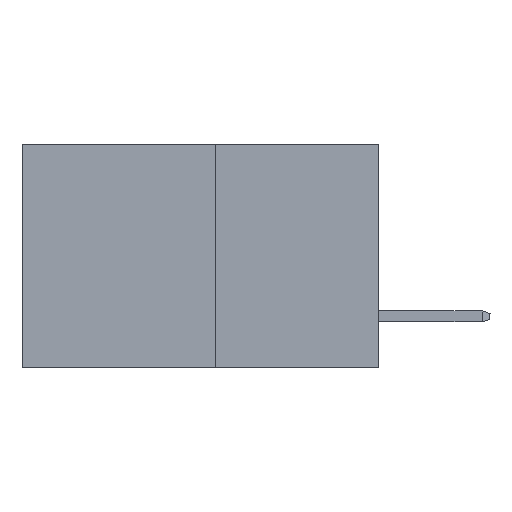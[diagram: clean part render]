
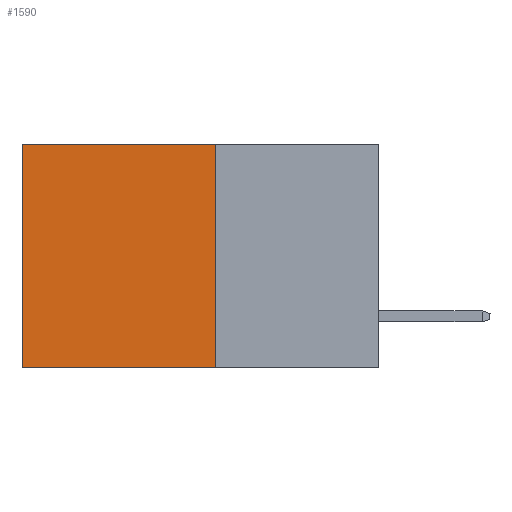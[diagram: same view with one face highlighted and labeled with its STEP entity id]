
A CAD part, left-side view. The second image highlights one B-rep face of the part: STEP entity #1590.
In plain terms, the highlighted planar face has unit normal (-1, 0, 0).
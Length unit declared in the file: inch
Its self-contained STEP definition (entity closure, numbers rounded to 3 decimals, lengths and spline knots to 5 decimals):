
#270 = EDGE_LOOP ( 'NONE', ( #2695, #4036, #4629, #5521 ) ) ;
#367 = EDGE_CURVE ( 'NONE', #10174, #7396, #2030, .T. ) ;
#636 = CARTESIAN_POINT ( 'NONE',  ( 0.277, 0.59, 0. ) ) ;
#1110 = LINE ( 'NONE', #10326, #13422 ) ;
#1590 = ADVANCED_FACE ( 'NONE', ( #10396 ), #5309, .F. ) ;
#2030 = LINE ( 'NONE', #9918, #14186 ) ;
#2095 = DIRECTION ( 'NONE',  ( 1., 0., 0. ) ) ;
#2695 = ORIENTED_EDGE ( 'NONE', *, *, #14201, .T. ) ;
#4036 = ORIENTED_EDGE ( 'NONE', *, *, #8668, .F. ) ;
#4629 = ORIENTED_EDGE ( 'NONE', *, *, #367, .F. ) ;
#5309 = PLANE ( 'NONE',  #12444 ) ;
#5311 = CARTESIAN_POINT ( 'NONE',  ( 0.277, 0.27, -0.37 ) ) ;
#5521 = ORIENTED_EDGE ( 'NONE', *, *, #14158, .T. ) ;
#5597 = CARTESIAN_POINT ( 'NONE',  ( 0.277, 0.27, 0. ) ) ;
#5866 = CARTESIAN_POINT ( 'NONE',  ( 0.277, 0.27, 0. ) ) ;
#6888 = LINE ( 'NONE', #9429, #12684 ) ;
#7340 = CARTESIAN_POINT ( 'NONE',  ( 0.277, 0.27, -0.37 ) ) ;
#7396 = VERTEX_POINT ( 'NONE', #7340 ) ;
#7897 = VERTEX_POINT ( 'NONE', #8015 ) ;
#8015 = CARTESIAN_POINT ( 'NONE',  ( 0.277, 0.59, -0.37 ) ) ;
#8668 = EDGE_CURVE ( 'NONE', #7396, #7897, #1110, .T. ) ;
#9429 = CARTESIAN_POINT ( 'NONE',  ( 0.277, 0.59, -0.37 ) ) ;
#9721 = VERTEX_POINT ( 'NONE', #636 ) ;
#9918 = CARTESIAN_POINT ( 'NONE',  ( 0.277, 0.27, -0.37 ) ) ;
#10174 = VERTEX_POINT ( 'NONE', #5597 ) ;
#10244 = DIRECTION ( 'NONE',  ( 0., 1., 0. ) ) ;
#10326 = CARTESIAN_POINT ( 'NONE',  ( 0.277, 0.27, -0.37 ) ) ;
#10396 = FACE_OUTER_BOUND ( 'NONE', #270, .T. ) ;
#10576 = DIRECTION ( 'NONE',  ( 0., 0., -1. ) ) ;
#10686 = LINE ( 'NONE', #5866, #13761 ) ;
#12444 = AXIS2_PLACEMENT_3D ( 'NONE', #5311, #2095, #14795 ) ;
#12684 = VECTOR ( 'NONE', #10576, 39.37008 ) ;
#13422 = VECTOR ( 'NONE', #10244, 39.37008 ) ;
#13498 = DIRECTION ( 'NONE',  ( 0., 0., -1. ) ) ;
#13761 = VECTOR ( 'NONE', #13946, 39.37008 ) ;
#13946 = DIRECTION ( 'NONE',  ( 0., 1., 0. ) ) ;
#14158 = EDGE_CURVE ( 'NONE', #10174, #9721, #10686, .T. ) ;
#14186 = VECTOR ( 'NONE', #13498, 39.37008 ) ;
#14201 = EDGE_CURVE ( 'NONE', #9721, #7897, #6888, .T. ) ;
#14795 = DIRECTION ( 'NONE',  ( 0., 0., -1. ) ) ;
